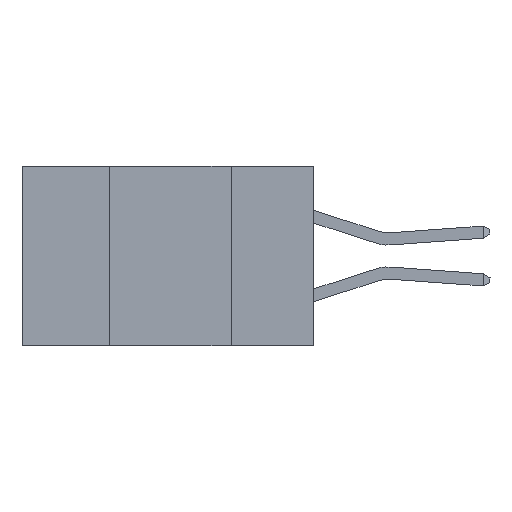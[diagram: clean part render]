
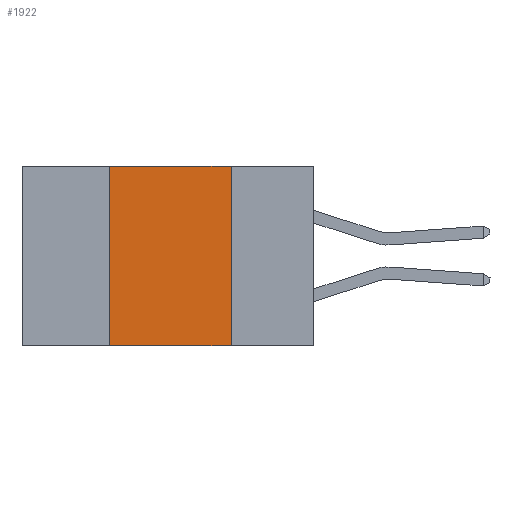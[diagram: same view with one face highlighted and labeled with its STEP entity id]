
A CAD part, left-side view. The second image highlights one B-rep face of the part: STEP entity #1922.
In plain terms, the highlighted planar face has unit normal (-1, 0, 0).
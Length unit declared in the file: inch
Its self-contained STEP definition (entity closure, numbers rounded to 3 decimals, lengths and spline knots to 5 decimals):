
#1406 = DIRECTION ( 'NONE',  ( 0., 0., -1. ) ) ;
#1922 = ADVANCED_FACE ( 'NONE', ( #29589 ), #10123, .F. ) ;
#2604 = DIRECTION ( 'NONE',  ( 0., 0., -1. ) ) ;
#4281 = DIRECTION ( 'NONE',  ( 0., 0., 1. ) ) ;
#6845 = EDGE_CURVE ( 'NONE', #6995, #10720, #7534, .T. ) ;
#6995 = VERTEX_POINT ( 'NONE', #13655 ) ;
#7095 = EDGE_CURVE ( 'NONE', #24324, #10720, #29481, .T. ) ;
#7534 = LINE ( 'NONE', #29765, #20832 ) ;
#8097 = ORIENTED_EDGE ( 'NONE', *, *, #6845, .F. ) ;
#9396 = EDGE_LOOP ( 'NONE', ( #8097, #22296, #12055, #25197 ) ) ;
#10123 = PLANE ( 'NONE',  #21685 ) ;
#10720 = VERTEX_POINT ( 'NONE', #13828 ) ;
#11019 = LINE ( 'NONE', #26773, #30255 ) ;
#12055 = ORIENTED_EDGE ( 'NONE', *, *, #21120, .F. ) ;
#12521 = CARTESIAN_POINT ( 'NONE',  ( 0., 0.6, 0. ) ) ;
#13010 = EDGE_CURVE ( 'NONE', #18443, #6995, #11019, .T. ) ;
#13655 = CARTESIAN_POINT ( 'NONE',  ( 0., 0.17, 0. ) ) ;
#13828 = CARTESIAN_POINT ( 'NONE',  ( 0., 0.17, -0.37 ) ) ;
#16857 = CARTESIAN_POINT ( 'NONE',  ( 0., 0.42, 0. ) ) ;
#18184 = DIRECTION ( 'NONE',  ( 0., -1., 0. ) ) ;
#18186 = LINE ( 'NONE', #16857, #29576 ) ;
#18443 = VERTEX_POINT ( 'NONE', #29521 ) ;
#19564 = DIRECTION ( 'NONE',  ( 0., -1., 0. ) ) ;
#20832 = VECTOR ( 'NONE', #1406, 39.37008 ) ;
#21120 = EDGE_CURVE ( 'NONE', #24324, #18443, #18186, .T. ) ;
#21685 = AXIS2_PLACEMENT_3D ( 'NONE', #12521, #29979, #2604 ) ;
#21854 = CARTESIAN_POINT ( 'NONE',  ( 0., 0.42, -0.37 ) ) ;
#22296 = ORIENTED_EDGE ( 'NONE', *, *, #13010, .F. ) ;
#23485 = CARTESIAN_POINT ( 'NONE',  ( 0., 0.6, -0.37 ) ) ;
#24324 = VERTEX_POINT ( 'NONE', #21854 ) ;
#25197 = ORIENTED_EDGE ( 'NONE', *, *, #7095, .T. ) ;
#26773 = CARTESIAN_POINT ( 'NONE',  ( 0., 0.6, 0. ) ) ;
#29481 = LINE ( 'NONE', #23485, #30242 ) ;
#29521 = CARTESIAN_POINT ( 'NONE',  ( 0., 0.42, 0. ) ) ;
#29576 = VECTOR ( 'NONE', #4281, 39.37008 ) ;
#29589 = FACE_OUTER_BOUND ( 'NONE', #9396, .T. ) ;
#29765 = CARTESIAN_POINT ( 'NONE',  ( 0., 0.17, 0. ) ) ;
#29979 = DIRECTION ( 'NONE',  ( 1., 0., 0. ) ) ;
#30242 = VECTOR ( 'NONE', #18184, 39.37008 ) ;
#30255 = VECTOR ( 'NONE', #19564, 39.37008 ) ;
